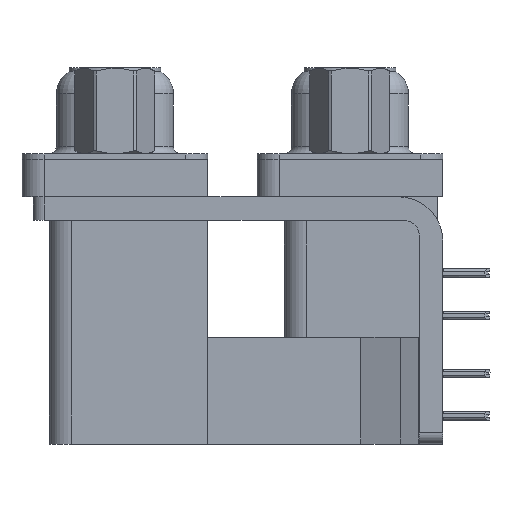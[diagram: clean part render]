
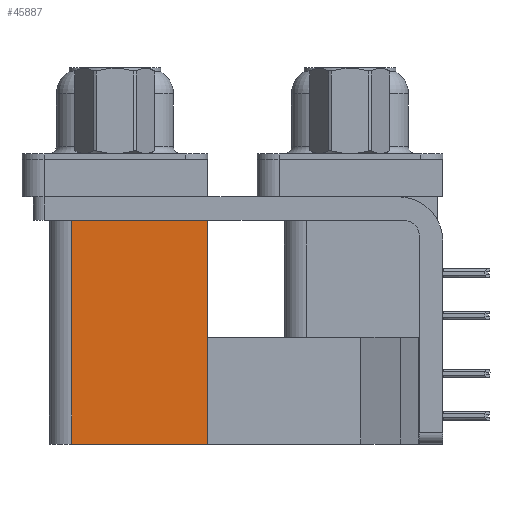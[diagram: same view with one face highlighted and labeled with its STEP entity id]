
A CAD part, left-side view. The second image highlights one B-rep face of the part: STEP entity #45887.
In plain terms, the highlighted planar face has unit normal (-1, 0, 0).
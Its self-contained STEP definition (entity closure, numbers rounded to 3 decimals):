
#307 = VERTEX_POINT ( 'NONE', #14116 ) ;
#3426 = CARTESIAN_POINT ( 'NONE',  ( 3.79, 18.8, -2.5 ) ) ;
#7173 = VERTEX_POINT ( 'NONE', #3426 ) ;
#8105 = VECTOR ( 'NONE', #23147, 1000. ) ;
#8536 = EDGE_CURVE ( 'NONE', #13520, #7173, #43453, .T. ) ;
#8934 = DIRECTION ( 'NONE',  ( 0., 1., 0. ) ) ;
#10769 = ORIENTED_EDGE ( 'NONE', *, *, #14814, .T. ) ;
#13085 = DIRECTION ( 'NONE',  ( 0., 1., 0. ) ) ;
#13520 = VERTEX_POINT ( 'NONE', #34960 ) ;
#14116 = CARTESIAN_POINT ( 'NONE',  ( 3.79, 9.6, -19.2 ) ) ;
#14814 = EDGE_CURVE ( 'NONE', #16818, #7173, #19749, .T. ) ;
#14889 = ORIENTED_EDGE ( 'NONE', *, *, #8536, .F. ) ;
#16116 = CARTESIAN_POINT ( 'NONE',  ( 3.79, 9.6, -19.2 ) ) ;
#16338 = DIRECTION ( 'NONE',  ( 0., 1., 0. ) ) ;
#16469 = VECTOR ( 'NONE', #8934, 1000. ) ;
#16577 = PLANE ( 'NONE',  #43909 ) ;
#16818 = VERTEX_POINT ( 'NONE', #25492 ) ;
#19749 = LINE ( 'NONE', #42246, #24256 ) ;
#19863 = LINE ( 'NONE', #34557, #16469 ) ;
#21302 = EDGE_LOOP ( 'NONE', ( #10769, #14889, #25304, #24924 ) ) ;
#22098 = DIRECTION ( 'NONE',  ( 0., 0., 1. ) ) ;
#23147 = DIRECTION ( 'NONE',  ( 0., 0., 1. ) ) ;
#23396 = CARTESIAN_POINT ( 'NONE',  ( 3.79, 9.6, -19.2 ) ) ;
#24256 = VECTOR ( 'NONE', #13085, 1000. ) ;
#24924 = ORIENTED_EDGE ( 'NONE', *, *, #43044, .T. ) ;
#25185 = CARTESIAN_POINT ( 'NONE',  ( 3.79, 18.8, -19.2 ) ) ;
#25304 = ORIENTED_EDGE ( 'NONE', *, *, #25647, .F. ) ;
#25492 = CARTESIAN_POINT ( 'NONE',  ( 3.79, 9.6, -2.5 ) ) ;
#25647 = EDGE_CURVE ( 'NONE', #307, #13520, #19863, .T. ) ;
#34557 = CARTESIAN_POINT ( 'NONE',  ( 3.79, 9.6, -19.2 ) ) ;
#34960 = CARTESIAN_POINT ( 'NONE',  ( 3.79, 18.8, -19.2 ) ) ;
#38628 = DIRECTION ( 'NONE',  ( 1., 0., 0. ) ) ;
#40693 = VECTOR ( 'NONE', #22098, 1000. ) ;
#42246 = CARTESIAN_POINT ( 'NONE',  ( 3.79, 9.6, -2.5 ) ) ;
#43044 = EDGE_CURVE ( 'NONE', #307, #16818, #45203, .T. ) ;
#43453 = LINE ( 'NONE', #25185, #40693 ) ;
#43864 = FACE_OUTER_BOUND ( 'NONE', #21302, .T. ) ;
#43909 = AXIS2_PLACEMENT_3D ( 'NONE', #16116, #38628, #16338 ) ;
#45203 = LINE ( 'NONE', #23396, #8105 ) ;
#45887 = ADVANCED_FACE ( 'NONE', ( #43864 ), #16577, .F. ) ;
